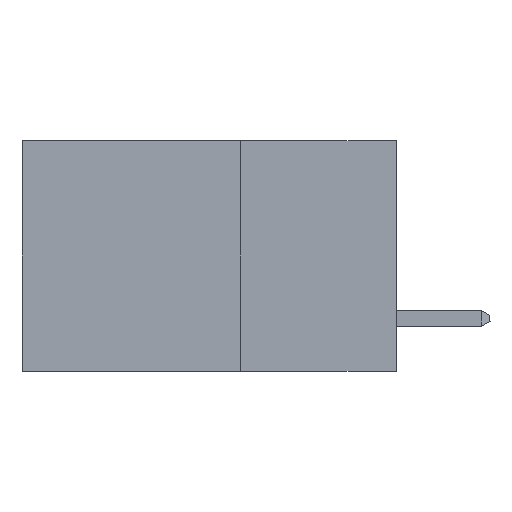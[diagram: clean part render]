
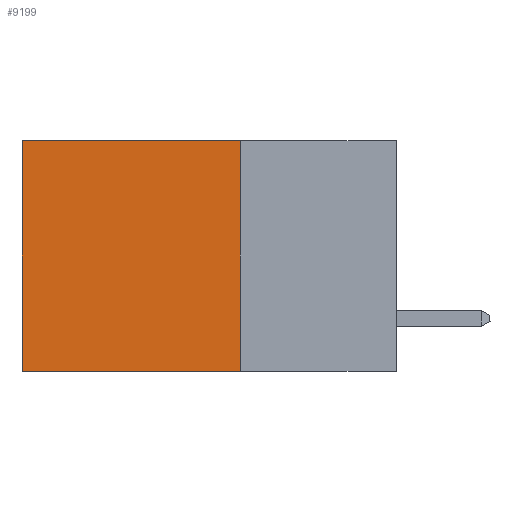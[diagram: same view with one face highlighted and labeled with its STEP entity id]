
A CAD part, left-side view. The second image highlights one B-rep face of the part: STEP entity #9199.
In plain terms, the highlighted planar face has unit normal (-1, 0, 0).
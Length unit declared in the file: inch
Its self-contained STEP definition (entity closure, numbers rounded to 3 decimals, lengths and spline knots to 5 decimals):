
#360 = LINE ( 'NONE', #18192, #917 ) ;
#544 = CARTESIAN_POINT ( 'NONE',  ( 0.298, 0.6, 0. ) ) ;
#917 = VECTOR ( 'NONE', #3413, 39.37008 ) ;
#1875 = CARTESIAN_POINT ( 'NONE',  ( 0.298, 0.25, 0. ) ) ;
#2926 = CARTESIAN_POINT ( 'NONE',  ( 0.298, 0.25, 0. ) ) ;
#2967 = LINE ( 'NONE', #21158, #7076 ) ;
#3413 = DIRECTION ( 'NONE',  ( 0., 0., -1. ) ) ;
#3661 = DIRECTION ( 'NONE',  ( 0., 0., -1. ) ) ;
#4838 = EDGE_CURVE ( 'NONE', #7248, #10120, #6890, .T. ) ;
#4967 = VECTOR ( 'NONE', #3661, 39.37008 ) ;
#5233 = FACE_OUTER_BOUND ( 'NONE', #17979, .T. ) ;
#5883 = ORIENTED_EDGE ( 'NONE', *, *, #4838, .F. ) ;
#6890 = LINE ( 'NONE', #19169, #18730 ) ;
#7076 = VECTOR ( 'NONE', #18047, 39.37008 ) ;
#7248 = VERTEX_POINT ( 'NONE', #11347 ) ;
#7526 = PLANE ( 'NONE',  #12827 ) ;
#9118 = CARTESIAN_POINT ( 'NONE',  ( 0.298, 0.25, 0. ) ) ;
#9197 = DIRECTION ( 'NONE',  ( 0., 0., -1. ) ) ;
#9199 = ADVANCED_FACE ( 'NONE', ( #5233 ), #7526, .F. ) ;
#10120 = VERTEX_POINT ( 'NONE', #16199 ) ;
#10730 = EDGE_CURVE ( 'NONE', #16993, #10120, #360, .T. ) ;
#11347 = CARTESIAN_POINT ( 'NONE',  ( 0.298, 0.25, -0.37 ) ) ;
#12669 = EDGE_CURVE ( 'NONE', #13068, #7248, #17690, .T. ) ;
#12827 = AXIS2_PLACEMENT_3D ( 'NONE', #9118, #18789, #9197 ) ;
#13068 = VERTEX_POINT ( 'NONE', #2926 ) ;
#13180 = EDGE_CURVE ( 'NONE', #13068, #16993, #2967, .T. ) ;
#14433 = DIRECTION ( 'NONE',  ( 0., 1., 0. ) ) ;
#16199 = CARTESIAN_POINT ( 'NONE',  ( 0.298, 0.6, -0.37 ) ) ;
#16661 = ORIENTED_EDGE ( 'NONE', *, *, #13180, .T. ) ;
#16993 = VERTEX_POINT ( 'NONE', #544 ) ;
#17690 = LINE ( 'NONE', #1875, #4967 ) ;
#17979 = EDGE_LOOP ( 'NONE', ( #18276, #5883, #18416, #16661 ) ) ;
#18047 = DIRECTION ( 'NONE',  ( 0., 1., 0. ) ) ;
#18192 = CARTESIAN_POINT ( 'NONE',  ( 0.298, 0.6, 0. ) ) ;
#18276 = ORIENTED_EDGE ( 'NONE', *, *, #10730, .T. ) ;
#18416 = ORIENTED_EDGE ( 'NONE', *, *, #12669, .F. ) ;
#18730 = VECTOR ( 'NONE', #14433, 39.37008 ) ;
#18789 = DIRECTION ( 'NONE',  ( 1., 0., 0. ) ) ;
#19169 = CARTESIAN_POINT ( 'NONE',  ( 0.298, 0.25, -0.37 ) ) ;
#21158 = CARTESIAN_POINT ( 'NONE',  ( 0.298, 0.25, 0. ) ) ;
